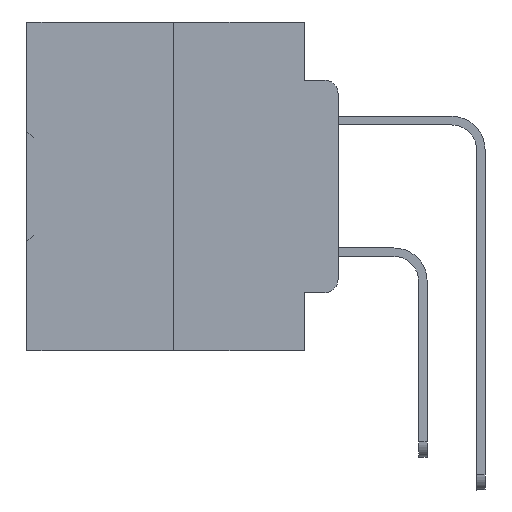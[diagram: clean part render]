
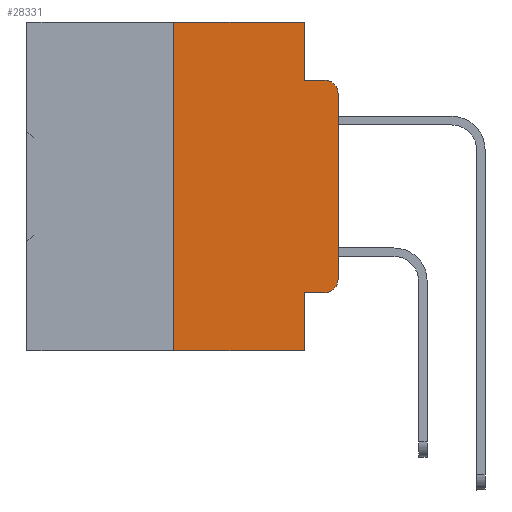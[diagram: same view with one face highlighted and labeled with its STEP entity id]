
A CAD part, left-side view. The second image highlights one B-rep face of the part: STEP entity #28331.
In plain terms, the highlighted planar face has unit normal (-1, 0, 0).
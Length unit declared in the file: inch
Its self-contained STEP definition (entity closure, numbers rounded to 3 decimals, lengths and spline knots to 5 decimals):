
#541 = VECTOR ( 'NONE', #10905, 39.37008 ) ;
#840 = AXIS2_PLACEMENT_3D ( 'NONE', #13847, #34453, #16869 ) ;
#1819 = LINE ( 'NONE', #36233, #29944 ) ;
#2358 = EDGE_LOOP ( 'NONE', ( #37416, #33347, #31291, #28371, #20558, #19230, #18775, #18814, #35797, #30247 ) ) ;
#3249 = DIRECTION ( 'NONE',  ( 0., -1., 0. ) ) ;
#4025 = CARTESIAN_POINT ( 'NONE',  ( 0., 0.25, 0. ) ) ;
#4034 = AXIS2_PLACEMENT_3D ( 'NONE', #13293, #31066, #13425 ) ;
#4880 = CARTESIAN_POINT ( 'NONE',  ( 0., 0.25, -0.5 ) ) ;
#5342 = VERTEX_POINT ( 'NONE', #32151 ) ;
#6015 = VERTEX_POINT ( 'NONE', #11856 ) ;
#6092 = CARTESIAN_POINT ( 'NONE',  ( 0., 0.051, -0.5 ) ) ;
#7109 = CARTESIAN_POINT ( 'NONE',  ( 0., 0.02, -0.4115 ) ) ;
#8259 = CARTESIAN_POINT ( 'NONE',  ( 0., 0.051, -0.4115 ) ) ;
#8452 = EDGE_CURVE ( 'NONE', #26979, #5342, #23602, .T. ) ;
#8706 = CARTESIAN_POINT ( 'NONE',  ( 0., 0., 0. ) ) ;
#9216 = EDGE_CURVE ( 'NONE', #21190, #26979, #29046, .T. ) ;
#9411 = LINE ( 'NONE', #17081, #19348 ) ;
#9436 = VERTEX_POINT ( 'NONE', #34628 ) ;
#9458 = VERTEX_POINT ( 'NONE', #4880 ) ;
#9510 = VERTEX_POINT ( 'NONE', #20252 ) ;
#10361 = PLANE ( 'NONE',  #4034 ) ;
#10905 = DIRECTION ( 'NONE',  ( 0., 0., 1. ) ) ;
#11856 = CARTESIAN_POINT ( 'NONE',  ( 0., 0.051, -0.0885 ) ) ;
#12536 = CARTESIAN_POINT ( 'NONE',  ( 0., 0.473, -0.5 ) ) ;
#12874 = CARTESIAN_POINT ( 'NONE',  ( 0., 0.051, -0.0885 ) ) ;
#13293 = CARTESIAN_POINT ( 'NONE',  ( 0., 0.473, 0. ) ) ;
#13425 = DIRECTION ( 'NONE',  ( 0., 0., -1. ) ) ;
#13847 = CARTESIAN_POINT ( 'NONE',  ( 0., 0.02, -0.1085 ) ) ;
#14166 = EDGE_CURVE ( 'NONE', #25109, #9436, #28918, .T. ) ;
#15153 = LINE ( 'NONE', #12874, #22993 ) ;
#15792 = VECTOR ( 'NONE', #26594, 39.37008 ) ;
#15873 = DIRECTION ( 'NONE',  ( -1., 0., 0. ) ) ;
#16286 = DIRECTION ( 'NONE',  ( 0., -1., 0. ) ) ;
#16869 = DIRECTION ( 'NONE',  ( 0., 0., -1. ) ) ;
#17081 = CARTESIAN_POINT ( 'NONE',  ( 0., 0.051, 0. ) ) ;
#17367 = EDGE_CURVE ( 'NONE', #33936, #21190, #27743, .T. ) ;
#18775 = ORIENTED_EDGE ( 'NONE', *, *, #23043, .T. ) ;
#18814 = ORIENTED_EDGE ( 'NONE', *, *, #19356, .F. ) ;
#19230 = ORIENTED_EDGE ( 'NONE', *, *, #21312, .F. ) ;
#19348 = VECTOR ( 'NONE', #22972, 39.37008 ) ;
#19356 = EDGE_CURVE ( 'NONE', #33936, #28750, #9411, .T. ) ;
#19990 = VECTOR ( 'NONE', #16286, 39.37008 ) ;
#20252 = CARTESIAN_POINT ( 'NONE',  ( 0., 0.02, -0.0885 ) ) ;
#20558 = ORIENTED_EDGE ( 'NONE', *, *, #14166, .F. ) ;
#21190 = VERTEX_POINT ( 'NONE', #7109 ) ;
#21312 = EDGE_CURVE ( 'NONE', #9458, #25109, #30597, .T. ) ;
#21595 = DIRECTION ( 'NONE',  ( 0., 0., -1. ) ) ;
#22972 = DIRECTION ( 'NONE',  ( 0., 0., -1. ) ) ;
#22993 = VECTOR ( 'NONE', #33498, 39.37008 ) ;
#23043 = EDGE_CURVE ( 'NONE', #9458, #28750, #28638, .T. ) ;
#23503 = AXIS2_PLACEMENT_3D ( 'NONE', #33469, #15873, #36448 ) ;
#23602 = LINE ( 'NONE', #8706, #15792 ) ;
#24194 = CIRCLE ( 'NONE', #840, 0.02 ) ;
#25109 = VERTEX_POINT ( 'NONE', #4025 ) ;
#25757 = DIRECTION ( 'NONE',  ( 0., -1., 0. ) ) ;
#26594 = DIRECTION ( 'NONE',  ( 0., 0., 1. ) ) ;
#26962 = FACE_OUTER_BOUND ( 'NONE', #2358, .T. ) ;
#26979 = VERTEX_POINT ( 'NONE', #38142 ) ;
#27743 = LINE ( 'NONE', #33866, #19990 ) ;
#27997 = VECTOR ( 'NONE', #25757, 39.37008 ) ;
#28331 = ADVANCED_FACE ( 'NONE', ( #26962 ), #10361, .F. ) ;
#28371 = ORIENTED_EDGE ( 'NONE', *, *, #31129, .F. ) ;
#28638 = LINE ( 'NONE', #12536, #36483 ) ;
#28684 = CARTESIAN_POINT ( 'NONE',  ( 0., 0.473, 0. ) ) ;
#28750 = VERTEX_POINT ( 'NONE', #6092 ) ;
#28918 = LINE ( 'NONE', #28684, #27997 ) ;
#29046 = CIRCLE ( 'NONE', #23503, 0.02 ) ;
#29944 = VECTOR ( 'NONE', #21595, 39.37008 ) ;
#30247 = ORIENTED_EDGE ( 'NONE', *, *, #9216, .T. ) ;
#30597 = LINE ( 'NONE', #31582, #541 ) ;
#31066 = DIRECTION ( 'NONE',  ( 1., 0., 0. ) ) ;
#31129 = EDGE_CURVE ( 'NONE', #9436, #6015, #1819, .T. ) ;
#31291 = ORIENTED_EDGE ( 'NONE', *, *, #33097, .F. ) ;
#31582 = CARTESIAN_POINT ( 'NONE',  ( 0., 0.25, 0. ) ) ;
#32151 = CARTESIAN_POINT ( 'NONE',  ( 0., 0., -0.1085 ) ) ;
#33097 = EDGE_CURVE ( 'NONE', #6015, #9510, #15153, .T. ) ;
#33347 = ORIENTED_EDGE ( 'NONE', *, *, #35081, .T. ) ;
#33469 = CARTESIAN_POINT ( 'NONE',  ( 0., 0.02, -0.3915 ) ) ;
#33498 = DIRECTION ( 'NONE',  ( 0., -1., 0. ) ) ;
#33866 = CARTESIAN_POINT ( 'NONE',  ( 0., 0.051, -0.4115 ) ) ;
#33936 = VERTEX_POINT ( 'NONE', #8259 ) ;
#34453 = DIRECTION ( 'NONE',  ( -1., 0., 0. ) ) ;
#34628 = CARTESIAN_POINT ( 'NONE',  ( 0., 0.051, 0. ) ) ;
#35081 = EDGE_CURVE ( 'NONE', #5342, #9510, #24194, .T. ) ;
#35797 = ORIENTED_EDGE ( 'NONE', *, *, #17367, .T. ) ;
#36233 = CARTESIAN_POINT ( 'NONE',  ( 0., 0.051, 0. ) ) ;
#36448 = DIRECTION ( 'NONE',  ( 0., 0., -1. ) ) ;
#36483 = VECTOR ( 'NONE', #3249, 39.37008 ) ;
#37416 = ORIENTED_EDGE ( 'NONE', *, *, #8452, .T. ) ;
#38142 = CARTESIAN_POINT ( 'NONE',  ( 0., 0., -0.3915 ) ) ;
